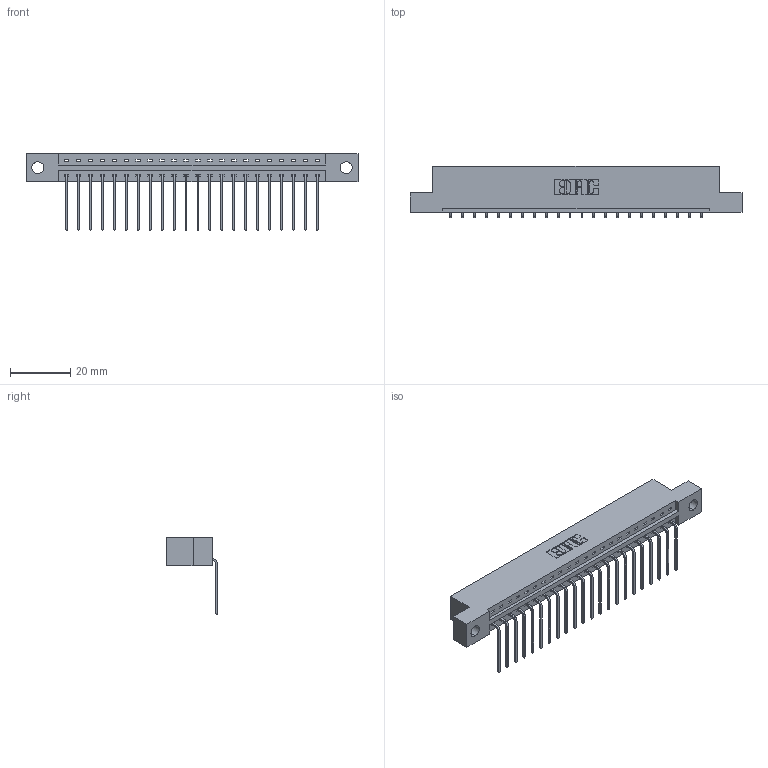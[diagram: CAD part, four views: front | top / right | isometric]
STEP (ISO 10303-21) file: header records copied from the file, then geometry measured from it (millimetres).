
FILE_DESCRIPTION (( 'STEP AP203' ), '1' );
FILE_NAME ('337-022-559-104.STEP', '2019-09-30T14:05:12', ( '' ), ( '' ), 'SwSTEP 2.0', 'SolidWorks 2016', '' );
FILE_SCHEMA (( 'CONFIG_CONTROL_DESIGN' ));
Length unit declared in the file: inch
Products named in the file (3): 337 Part_Flush Mounting Lugs - 0.156 Dia-TH; 345-292-001_558 559 Tail - 1; 337-022-559-104
Assembly tree (23 placements, depth 2):
  337-022-559-104
    337 Part_Flush Mounting Lugs - 0.156 Dia-TH
    345-292-001_558 559 Tail - 1  x22
Bounding box: 110.19 x 17.09 x 25.53 mm (x, y, z)
Volume: 11187.1 mm3; surface area: 11694.8 mm2
Topology: 23 solids, 23 shells, 1522 faces, 4579 edges, 3022 vertices
Faces by surface type: plane 1126, cylinder 396
Entity records: 19027 total; most frequent: CARTESIAN_POINT 3320, ORIENTED_EDGE 3278, DIRECTION 2835, EDGE_CURVE 1639, VECTOR 1511, LINE 1511, VERTEX_POINT 1090, AXIS2_PLACEMENT_3D 662
